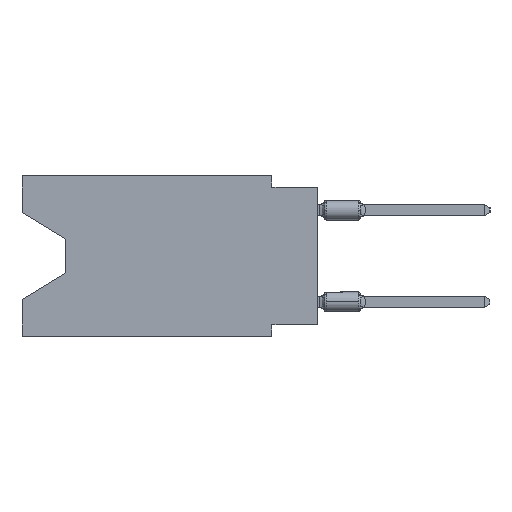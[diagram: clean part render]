
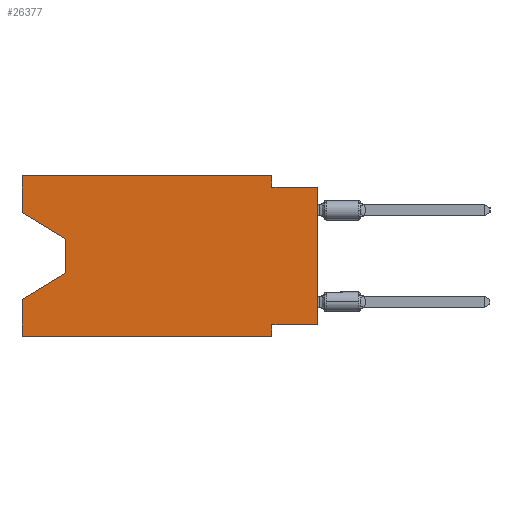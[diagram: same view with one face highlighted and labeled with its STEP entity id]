
A CAD part, left-side view. The second image highlights one B-rep face of the part: STEP entity #26377.
In plain terms, the highlighted planar face has unit normal (-1, 0, 0).
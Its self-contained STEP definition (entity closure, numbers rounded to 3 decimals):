
#1997 = CARTESIAN_POINT ( 'NONE',  ( 0., 16.383, -2.038 ) ) ;
#2740 = DIRECTION ( 'NONE',  ( 0., -0.855, -0.519 ) ) ;
#3287 = CARTESIAN_POINT ( 'NONE',  ( 0., 13.97, -3.505 ) ) ;
#3428 = CARTESIAN_POINT ( 'NONE',  ( 0., 16.383, -2.038 ) ) ;
#4945 = EDGE_CURVE ( 'NONE', #33139, #14285, #7890, .T. ) ;
#5039 = DIRECTION ( 'NONE',  ( 0., 0., 1. ) ) ;
#6423 = CARTESIAN_POINT ( 'NONE',  ( 0., 16.383, -8.89 ) ) ;
#7132 = ORIENTED_EDGE ( 'NONE', *, *, #53499, .F. ) ;
#7890 = LINE ( 'NONE', #12424, #66876 ) ;
#8373 = PLANE ( 'NONE',  #64500 ) ;
#8962 = CARTESIAN_POINT ( 'NONE',  ( 0., 0., -0.635 ) ) ;
#9610 = CARTESIAN_POINT ( 'NONE',  ( 0., 16.383, 0. ) ) ;
#9655 = ORIENTED_EDGE ( 'NONE', *, *, #40450, .F. ) ;
#10318 = DIRECTION ( 'NONE',  ( 0., 0.855, -0.519 ) ) ;
#10816 = VECTOR ( 'NONE', #37522, 1000. ) ;
#11652 = CARTESIAN_POINT ( 'NONE',  ( 0., 0., -8.255 ) ) ;
#12424 = CARTESIAN_POINT ( 'NONE',  ( 0., 2.54, -8.89 ) ) ;
#12988 = CARTESIAN_POINT ( 'NONE',  ( 0., 2.54, -8.255 ) ) ;
#14285 = VERTEX_POINT ( 'NONE', #59859 ) ;
#14712 = VERTEX_POINT ( 'NONE', #6423 ) ;
#18877 = VERTEX_POINT ( 'NONE', #29681 ) ;
#19157 = CARTESIAN_POINT ( 'NONE',  ( 0., 16.383, 0. ) ) ;
#20624 = EDGE_CURVE ( 'NONE', #62196, #50305, #31535, .T. ) ;
#21347 = LINE ( 'NONE', #42613, #37703 ) ;
#22336 = CARTESIAN_POINT ( 'NONE',  ( 0., 2.54, -0.635 ) ) ;
#22739 = LINE ( 'NONE', #54134, #68429 ) ;
#22819 = VECTOR ( 'NONE', #38517, 1000. ) ;
#24460 = VERTEX_POINT ( 'NONE', #3287 ) ;
#25645 = ORIENTED_EDGE ( 'NONE', *, *, #20624, .F. ) ;
#25997 = ORIENTED_EDGE ( 'NONE', *, *, #51934, .T. ) ;
#26028 = VECTOR ( 'NONE', #2740, 1000. ) ;
#26369 = CARTESIAN_POINT ( 'NONE',  ( 0., 13.97, -5.385 ) ) ;
#26377 = ADVANCED_FACE ( 'NONE', ( #46034 ), #8373, .F. ) ;
#27634 = DIRECTION ( 'NONE',  ( 0., -1., 0. ) ) ;
#28086 = DIRECTION ( 'NONE',  ( 0., 0., -1. ) ) ;
#29176 = DIRECTION ( 'NONE',  ( 0., 0., -1. ) ) ;
#29681 = CARTESIAN_POINT ( 'NONE',  ( 0., 13.97, -5.385 ) ) ;
#30992 = EDGE_CURVE ( 'NONE', #14712, #43517, #21347, .T. ) ;
#31256 = DIRECTION ( 'NONE',  ( 0., 0., -1. ) ) ;
#31535 = LINE ( 'NONE', #52809, #44070 ) ;
#32195 = ORIENTED_EDGE ( 'NONE', *, *, #37622, .T. ) ;
#33139 = VERTEX_POINT ( 'NONE', #12988 ) ;
#33574 = CARTESIAN_POINT ( 'NONE',  ( 0., 2.54, 0. ) ) ;
#34854 = LINE ( 'NONE', #19157, #38165 ) ;
#35770 = ORIENTED_EDGE ( 'NONE', *, *, #4945, .F. ) ;
#36396 = ORIENTED_EDGE ( 'NONE', *, *, #37889, .F. ) ;
#36482 = CARTESIAN_POINT ( 'NONE',  ( 0., 2.54, 0. ) ) ;
#37166 = LINE ( 'NONE', #36482, #57140 ) ;
#37522 = DIRECTION ( 'NONE',  ( 0., -1., 0. ) ) ;
#37622 = EDGE_CURVE ( 'NONE', #62196, #24460, #41094, .T. ) ;
#37703 = VECTOR ( 'NONE', #58663, 1000. ) ;
#37889 = EDGE_CURVE ( 'NONE', #50305, #44635, #34854, .T. ) ;
#38165 = VECTOR ( 'NONE', #50208, 1000. ) ;
#38438 = EDGE_CURVE ( 'NONE', #44635, #45003, #37166, .T. ) ;
#38517 = DIRECTION ( 'NONE',  ( 0., 1., 0. ) ) ;
#39579 = LINE ( 'NONE', #49695, #44747 ) ;
#40276 = EDGE_CURVE ( 'NONE', #18877, #43517, #67876, .T. ) ;
#40450 = EDGE_CURVE ( 'NONE', #45003, #63473, #59476, .T. ) ;
#41094 = LINE ( 'NONE', #3428, #26028 ) ;
#42613 = CARTESIAN_POINT ( 'NONE',  ( 0., 16.383, 0. ) ) ;
#42808 = LINE ( 'NONE', #51736, #43479 ) ;
#43406 = LINE ( 'NONE', #11652, #22819 ) ;
#43479 = VECTOR ( 'NONE', #57309, 1000. ) ;
#43517 = VERTEX_POINT ( 'NONE', #50634 ) ;
#44070 = VECTOR ( 'NONE', #5039, 1000. ) ;
#44635 = VERTEX_POINT ( 'NONE', #33574 ) ;
#44732 = ORIENTED_EDGE ( 'NONE', *, *, #40276, .T. ) ;
#44747 = VECTOR ( 'NONE', #28086, 1000. ) ;
#45003 = VERTEX_POINT ( 'NONE', #22336 ) ;
#46034 = FACE_OUTER_BOUND ( 'NONE', #57911, .T. ) ;
#47612 = VERTEX_POINT ( 'NONE', #52952 ) ;
#49695 = CARTESIAN_POINT ( 'NONE',  ( 0., 13.97, -3.505 ) ) ;
#50208 = DIRECTION ( 'NONE',  ( 0., -1., 0. ) ) ;
#50305 = VERTEX_POINT ( 'NONE', #9610 ) ;
#50634 = CARTESIAN_POINT ( 'NONE',  ( 0., 16.383, -6.852 ) ) ;
#51736 = CARTESIAN_POINT ( 'NONE',  ( 0., 0., 0. ) ) ;
#51934 = EDGE_CURVE ( 'NONE', #14712, #14285, #22739, .T. ) ;
#52798 = EDGE_CURVE ( 'NONE', #47612, #63473, #42808, .T. ) ;
#52809 = CARTESIAN_POINT ( 'NONE',  ( 0., 16.383, 0. ) ) ;
#52952 = CARTESIAN_POINT ( 'NONE',  ( 0., 0., -8.255 ) ) ;
#53499 = EDGE_CURVE ( 'NONE', #47612, #33139, #43406, .T. ) ;
#54134 = CARTESIAN_POINT ( 'NONE',  ( 0., 16.383, -8.89 ) ) ;
#56226 = ORIENTED_EDGE ( 'NONE', *, *, #38438, .F. ) ;
#57140 = VECTOR ( 'NONE', #31256, 1000. ) ;
#57309 = DIRECTION ( 'NONE',  ( 0., 0., 1. ) ) ;
#57911 = EDGE_LOOP ( 'NONE', ( #32195, #60617, #44732, #58153, #25997, #35770, #7132, #59113, #9655, #56226, #36396, #25645 ) ) ;
#58153 = ORIENTED_EDGE ( 'NONE', *, *, #30992, .F. ) ;
#58449 = CARTESIAN_POINT ( 'NONE',  ( 0., 0., -0.635 ) ) ;
#58663 = DIRECTION ( 'NONE',  ( 0., 0., 1. ) ) ;
#59113 = ORIENTED_EDGE ( 'NONE', *, *, #52798, .T. ) ;
#59476 = LINE ( 'NONE', #58449, #10816 ) ;
#59859 = CARTESIAN_POINT ( 'NONE',  ( 0., 2.54, -8.89 ) ) ;
#60617 = ORIENTED_EDGE ( 'NONE', *, *, #62580, .T. ) ;
#61734 = DIRECTION ( 'NONE',  ( 1., 0., 0. ) ) ;
#62196 = VERTEX_POINT ( 'NONE', #1997 ) ;
#62580 = EDGE_CURVE ( 'NONE', #24460, #18877, #39579, .T. ) ;
#63144 = VECTOR ( 'NONE', #10318, 1000. ) ;
#63473 = VERTEX_POINT ( 'NONE', #8962 ) ;
#64500 = AXIS2_PLACEMENT_3D ( 'NONE', #67297, #61734, #66267 ) ;
#66267 = DIRECTION ( 'NONE',  ( 0., 0., -1. ) ) ;
#66876 = VECTOR ( 'NONE', #29176, 1000. ) ;
#67297 = CARTESIAN_POINT ( 'NONE',  ( 0., 16.383, 0. ) ) ;
#67876 = LINE ( 'NONE', #26369, #63144 ) ;
#68429 = VECTOR ( 'NONE', #27634, 1000. ) ;
